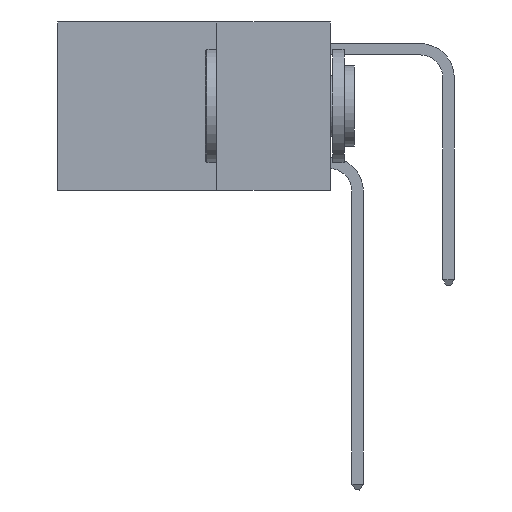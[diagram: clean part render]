
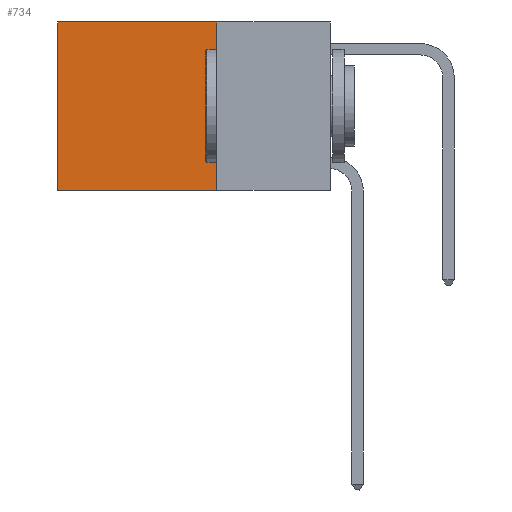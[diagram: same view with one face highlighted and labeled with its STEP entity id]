
A CAD part, left-side view. The second image highlights one B-rep face of the part: STEP entity #734.
In plain terms, the highlighted planar face has unit normal (-1, 0, 0).
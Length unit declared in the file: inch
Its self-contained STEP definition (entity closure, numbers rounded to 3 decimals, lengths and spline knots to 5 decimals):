
#247 = CARTESIAN_POINT ( 'NONE',  ( 0.2625, 0.25, 0. ) ) ;
#734 = ADVANCED_FACE ( 'NONE', ( #11456 ), #12436, .F. ) ;
#741 = CARTESIAN_POINT ( 'NONE',  ( 0.2625, 0.25, -0.37 ) ) ;
#2296 = DIRECTION ( 'NONE',  ( 1., 0., 0. ) ) ;
#2638 = VECTOR ( 'NONE', #5594, 39.37008 ) ;
#3127 = CARTESIAN_POINT ( 'NONE',  ( 0.2625, 0.6, -0.37 ) ) ;
#3439 = VERTEX_POINT ( 'NONE', #9538 ) ;
#3616 = EDGE_CURVE ( 'NONE', #9777, #21396, #23177, .T. ) ;
#4539 = EDGE_LOOP ( 'NONE', ( #15350, #5991, #25755, #5753 ) ) ;
#5594 = DIRECTION ( 'NONE',  ( 0., 1., 0. ) ) ;
#5753 = ORIENTED_EDGE ( 'NONE', *, *, #15436, .T. ) ;
#5991 = ORIENTED_EDGE ( 'NONE', *, *, #15000, .F. ) ;
#9538 = CARTESIAN_POINT ( 'NONE',  ( 0.2625, 0.25, 0. ) ) ;
#9777 = VERTEX_POINT ( 'NONE', #20237 ) ;
#10242 = CARTESIAN_POINT ( 'NONE',  ( 0.2625, 0.25, -0.37 ) ) ;
#11456 = FACE_OUTER_BOUND ( 'NONE', #4539, .T. ) ;
#12277 = DIRECTION ( 'NONE',  ( 0., 1., 0. ) ) ;
#12436 = PLANE ( 'NONE',  #16169 ) ;
#12856 = LINE ( 'NONE', #10242, #22983 ) ;
#13058 = VECTOR ( 'NONE', #22723, 39.37008 ) ;
#14789 = VECTOR ( 'NONE', #26250, 39.37008 ) ;
#14930 = EDGE_CURVE ( 'NONE', #3439, #23226, #15420, .T. ) ;
#15000 = EDGE_CURVE ( 'NONE', #23226, #21396, #12856, .T. ) ;
#15350 = ORIENTED_EDGE ( 'NONE', *, *, #3616, .T. ) ;
#15420 = LINE ( 'NONE', #24208, #14789 ) ;
#15436 = EDGE_CURVE ( 'NONE', #3439, #9777, #18839, .T. ) ;
#15734 = CARTESIAN_POINT ( 'NONE',  ( 0.2625, 0.25, 0. ) ) ;
#16169 = AXIS2_PLACEMENT_3D ( 'NONE', #247, #2296, #16537 ) ;
#16537 = DIRECTION ( 'NONE',  ( 0., 0., -1. ) ) ;
#18839 = LINE ( 'NONE', #15734, #2638 ) ;
#20237 = CARTESIAN_POINT ( 'NONE',  ( 0.2625, 0.6, 0. ) ) ;
#20689 = CARTESIAN_POINT ( 'NONE',  ( 0.2625, 0.6, 0. ) ) ;
#21396 = VERTEX_POINT ( 'NONE', #3127 ) ;
#22723 = DIRECTION ( 'NONE',  ( 0., 0., -1. ) ) ;
#22983 = VECTOR ( 'NONE', #12277, 39.37008 ) ;
#23177 = LINE ( 'NONE', #20689, #13058 ) ;
#23226 = VERTEX_POINT ( 'NONE', #741 ) ;
#24208 = CARTESIAN_POINT ( 'NONE',  ( 0.2625, 0.25, 0. ) ) ;
#25755 = ORIENTED_EDGE ( 'NONE', *, *, #14930, .F. ) ;
#26250 = DIRECTION ( 'NONE',  ( 0., 0., -1. ) ) ;
